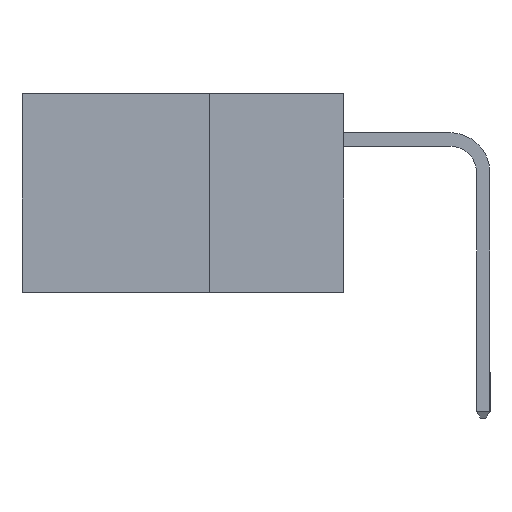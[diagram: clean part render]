
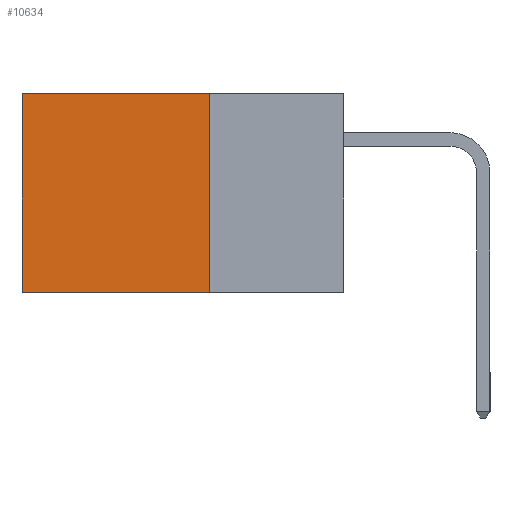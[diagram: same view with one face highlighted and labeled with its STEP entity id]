
A CAD part, left-side view. The second image highlights one B-rep face of the part: STEP entity #10634.
In plain terms, the highlighted planar face has unit normal (-1, 0, 0).
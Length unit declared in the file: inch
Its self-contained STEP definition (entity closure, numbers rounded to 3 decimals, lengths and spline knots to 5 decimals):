
#347 = EDGE_LOOP ( 'NONE', ( #6115, #3348, #3371, #11430 ) ) ;
#924 = CARTESIAN_POINT ( 'NONE',  ( 0.2615, 0.6, 0. ) ) ;
#1940 = CARTESIAN_POINT ( 'NONE',  ( 0.2615, 0.25, -0.37 ) ) ;
#2108 = DIRECTION ( 'NONE',  ( 0., 0., -1. ) ) ;
#2148 = VECTOR ( 'NONE', #13530, 39.37008 ) ;
#2652 = VECTOR ( 'NONE', #6201, 39.37008 ) ;
#3348 = ORIENTED_EDGE ( 'NONE', *, *, #5554, .F. ) ;
#3371 = ORIENTED_EDGE ( 'NONE', *, *, #5080, .F. ) ;
#4141 = CARTESIAN_POINT ( 'NONE',  ( 0.2615, 0.25, -0.37 ) ) ;
#4678 = VERTEX_POINT ( 'NONE', #6913 ) ;
#4816 = LINE ( 'NONE', #9757, #8220 ) ;
#5080 = EDGE_CURVE ( 'NONE', #10710, #7239, #9442, .T. ) ;
#5284 = CARTESIAN_POINT ( 'NONE',  ( 0.2615, 0.25, 0. ) ) ;
#5554 = EDGE_CURVE ( 'NONE', #7239, #4678, #11249, .T. ) ;
#5917 = EDGE_CURVE ( 'NONE', #9159, #4678, #4816, .T. ) ;
#6115 = ORIENTED_EDGE ( 'NONE', *, *, #5917, .T. ) ;
#6201 = DIRECTION ( 'NONE',  ( 0., 1., 0. ) ) ;
#6913 = CARTESIAN_POINT ( 'NONE',  ( 0.2615, 0.6, -0.37 ) ) ;
#7239 = VERTEX_POINT ( 'NONE', #4141 ) ;
#7586 = EDGE_CURVE ( 'NONE', #10710, #9159, #7752, .T. ) ;
#7752 = LINE ( 'NONE', #5284, #2148 ) ;
#8220 = VECTOR ( 'NONE', #12131, 39.37008 ) ;
#8463 = CARTESIAN_POINT ( 'NONE',  ( 0.2615, 0.25, 0. ) ) ;
#9159 = VERTEX_POINT ( 'NONE', #924 ) ;
#9442 = LINE ( 'NONE', #15351, #15025 ) ;
#9757 = CARTESIAN_POINT ( 'NONE',  ( 0.2615, 0.6, -0.37 ) ) ;
#10611 = DIRECTION ( 'NONE',  ( 1., 0., 0. ) ) ;
#10634 = ADVANCED_FACE ( 'NONE', ( #12460 ), #11626, .F. ) ;
#10710 = VERTEX_POINT ( 'NONE', #8463 ) ;
#11249 = LINE ( 'NONE', #12383, #2652 ) ;
#11336 = AXIS2_PLACEMENT_3D ( 'NONE', #1940, #10611, #11789 ) ;
#11430 = ORIENTED_EDGE ( 'NONE', *, *, #7586, .T. ) ;
#11626 = PLANE ( 'NONE',  #11336 ) ;
#11789 = DIRECTION ( 'NONE',  ( 0., 0., -1. ) ) ;
#12131 = DIRECTION ( 'NONE',  ( 0., 0., -1. ) ) ;
#12383 = CARTESIAN_POINT ( 'NONE',  ( 0.2615, 0.25, -0.37 ) ) ;
#12460 = FACE_OUTER_BOUND ( 'NONE', #347, .T. ) ;
#13530 = DIRECTION ( 'NONE',  ( 0., 1., 0. ) ) ;
#15025 = VECTOR ( 'NONE', #2108, 39.37008 ) ;
#15351 = CARTESIAN_POINT ( 'NONE',  ( 0.2615, 0.25, -0.37 ) ) ;
